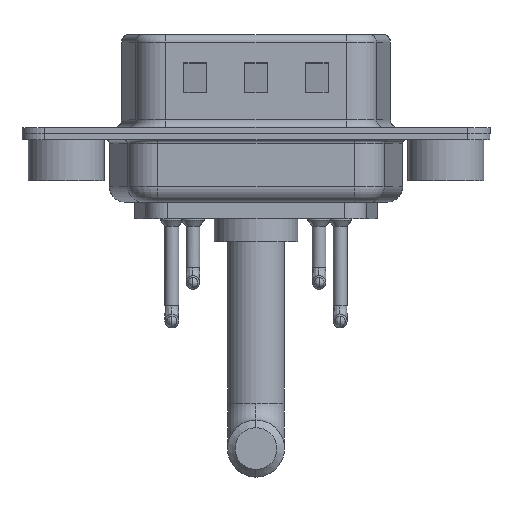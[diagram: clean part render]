
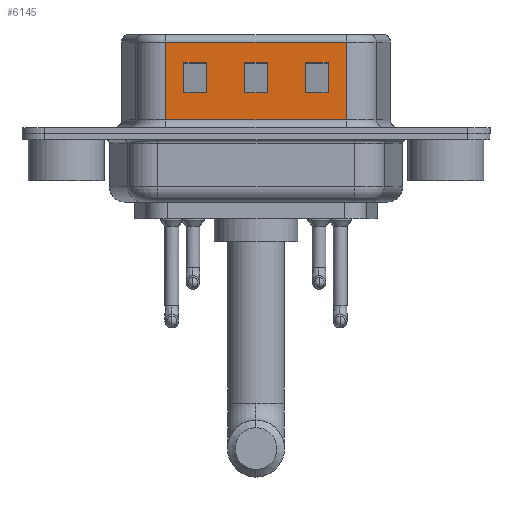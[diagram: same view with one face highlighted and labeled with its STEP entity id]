
A CAD part, front view. The second image highlights one B-rep face of the part: STEP entity #6145.
In plain terms, the highlighted planar face has unit normal (0, -1, 0).
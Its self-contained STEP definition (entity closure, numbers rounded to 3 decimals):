
#58 = VECTOR ( 'NONE', #6929, 1000. ) ;
#117 = AXIS2_PLACEMENT_3D ( 'NONE', #632, #735, #10937 ) ;
#134 = VECTOR ( 'NONE', #10615, 1000. ) ;
#245 = CARTESIAN_POINT ( 'NONE',  ( 18.451, -4.55, 6.02 ) ) ;
#406 = CARTESIAN_POINT ( 'NONE',  ( 13.25, -4.55, 4.705 ) ) ;
#409 = LINE ( 'NONE', #6395, #10310 ) ;
#414 = CARTESIAN_POINT ( 'NONE',  ( 6.549, -4.55, 0.9 ) ) ;
#632 = CARTESIAN_POINT ( 'NONE',  ( 18.451, -4.55, 6.52 ) ) ;
#735 = DIRECTION ( 'NONE',  ( 0., 1., 0. ) ) ;
#1160 = LINE ( 'NONE', #11468, #15240 ) ;
#1430 = ORIENTED_EDGE ( 'NONE', *, *, #16642, .T. ) ;
#1433 = EDGE_CURVE ( 'NONE', #14600, #17532, #16734, .T. ) ;
#1516 = CARTESIAN_POINT ( 'NONE',  ( 18.451, -4.55, 0.9 ) ) ;
#1538 = CARTESIAN_POINT ( 'NONE',  ( 13.25, -4.55, 6.52 ) ) ;
#1655 = EDGE_LOOP ( 'NONE', ( #2339, #8124, #1430, #2945 ) ) ;
#1727 = CARTESIAN_POINT ( 'NONE',  ( 22.451, -4.55, 4.705 ) ) ;
#1735 = DIRECTION ( 'NONE',  ( -1., 0., 0. ) ) ;
#1868 = VERTEX_POINT ( 'NONE', #414 ) ;
#2016 = PLANE ( 'NONE',  #117 ) ;
#2027 = EDGE_LOOP ( 'NONE', ( #11961, #11891, #10705, #10154 ) ) ;
#2086 = CARTESIAN_POINT ( 'NONE',  ( 11.75, -4.55, 2.705 ) ) ;
#2339 = ORIENTED_EDGE ( 'NONE', *, *, #18129, .T. ) ;
#2393 = CARTESIAN_POINT ( 'NONE',  ( 18.451, -4.55, 0.9 ) ) ;
#2700 = CARTESIAN_POINT ( 'NONE',  ( 15.75, -4.55, 4.705 ) ) ;
#2804 = CARTESIAN_POINT ( 'NONE',  ( 15.75, -4.55, 6.52 ) ) ;
#2911 = VERTEX_POINT ( 'NONE', #2700 ) ;
#2945 = ORIENTED_EDGE ( 'NONE', *, *, #7511, .T. ) ;
#3019 = VECTOR ( 'NONE', #12900, 1000. ) ;
#3133 = DIRECTION ( 'NONE',  ( 0., 0., 1. ) ) ;
#3438 = DIRECTION ( 'NONE',  ( 0., 0., 1. ) ) ;
#3482 = LINE ( 'NONE', #1727, #17855 ) ;
#3500 = EDGE_LOOP ( 'NONE', ( #7476, #10451, #7581, #7865 ) ) ;
#3657 = VERTEX_POINT ( 'NONE', #11320 ) ;
#3821 = EDGE_CURVE ( 'NONE', #17739, #10641, #14548, .T. ) ;
#3990 = VECTOR ( 'NONE', #15530, 1000. ) ;
#4045 = EDGE_CURVE ( 'NONE', #10447, #2911, #18175, .T. ) ;
#4546 = LINE ( 'NONE', #4635, #134 ) ;
#4635 = CARTESIAN_POINT ( 'NONE',  ( 17.25, -4.55, 6.52 ) ) ;
#4716 = VECTOR ( 'NONE', #1735, 1000. ) ;
#5061 = FACE_BOUND ( 'NONE', #3500, .T. ) ;
#5177 = CARTESIAN_POINT ( 'NONE',  ( 18.451, -4.55, 4.705 ) ) ;
#5260 = EDGE_CURVE ( 'NONE', #1868, #14274, #16618, .T. ) ;
#5423 = VERTEX_POINT ( 'NONE', #2086 ) ;
#6145 = ADVANCED_FACE ( 'NONE', ( #17207, #5061, #14047, #6521 ), #2016, .F. ) ;
#6224 = DIRECTION ( 'NONE',  ( 1., 0., 0. ) ) ;
#6346 = VERTEX_POINT ( 'NONE', #8486 ) ;
#6395 = CARTESIAN_POINT ( 'NONE',  ( 14.451, -4.55, 4.705 ) ) ;
#6442 = VERTEX_POINT ( 'NONE', #13268 ) ;
#6471 = EDGE_CURVE ( 'NONE', #18734, #11791, #4546, .T. ) ;
#6477 = VECTOR ( 'NONE', #3133, 1000. ) ;
#6521 = FACE_OUTER_BOUND ( 'NONE', #10357, .T. ) ;
#6570 = CARTESIAN_POINT ( 'NONE',  ( 15.75, -4.55, 2.705 ) ) ;
#6929 = DIRECTION ( 'NONE',  ( -1., 0., 0. ) ) ;
#7072 = EDGE_CURVE ( 'NONE', #10641, #16116, #12359, .T. ) ;
#7476 = ORIENTED_EDGE ( 'NONE', *, *, #6471, .T. ) ;
#7511 = EDGE_CURVE ( 'NONE', #5423, #6442, #9388, .T. ) ;
#7522 = DIRECTION ( 'NONE',  ( 0., 0., -1. ) ) ;
#7578 = ORIENTED_EDGE ( 'NONE', *, *, #5260, .T. ) ;
#7581 = ORIENTED_EDGE ( 'NONE', *, *, #4045, .T. ) ;
#7796 = DIRECTION ( 'NONE',  ( 1., 0., 0. ) ) ;
#7865 = ORIENTED_EDGE ( 'NONE', *, *, #14056, .T. ) ;
#7894 = LINE ( 'NONE', #9546, #16902 ) ;
#8124 = ORIENTED_EDGE ( 'NONE', *, *, #18319, .T. ) ;
#8486 = CARTESIAN_POINT ( 'NONE',  ( 9.25, -4.55, 4.705 ) ) ;
#8517 = LINE ( 'NONE', #1538, #13091 ) ;
#8553 = EDGE_CURVE ( 'NONE', #17532, #1868, #1160, .T. ) ;
#8679 = LINE ( 'NONE', #17796, #3019 ) ;
#8778 = DIRECTION ( 'NONE',  ( 0., 0., 1. ) ) ;
#8957 = ORIENTED_EDGE ( 'NONE', *, *, #8553, .T. ) ;
#9388 = LINE ( 'NONE', #15279, #6477 ) ;
#9546 = CARTESIAN_POINT ( 'NONE',  ( 18.451, -4.55, 6.52 ) ) ;
#9547 = CARTESIAN_POINT ( 'NONE',  ( 22.451, -4.55, 2.705 ) ) ;
#9673 = DIRECTION ( 'NONE',  ( 1., 0., 0. ) ) ;
#10154 = ORIENTED_EDGE ( 'NONE', *, *, #13076, .T. ) ;
#10310 = VECTOR ( 'NONE', #12368, 1000. ) ;
#10357 = EDGE_LOOP ( 'NONE', ( #10450, #15410, #8957, #7578 ) ) ;
#10447 = VERTEX_POINT ( 'NONE', #6570 ) ;
#10450 = ORIENTED_EDGE ( 'NONE', *, *, #14114, .F. ) ;
#10451 = ORIENTED_EDGE ( 'NONE', *, *, #18701, .T. ) ;
#10615 = DIRECTION ( 'NONE',  ( 0., 0., -1. ) ) ;
#10626 = CARTESIAN_POINT ( 'NONE',  ( 7.75, -4.55, 4.705 ) ) ;
#10641 = VERTEX_POINT ( 'NONE', #13114 ) ;
#10705 = ORIENTED_EDGE ( 'NONE', *, *, #7072, .T. ) ;
#10937 = DIRECTION ( 'NONE',  ( -1., 0., 0. ) ) ;
#11050 = VECTOR ( 'NONE', #6224, 1000. ) ;
#11095 = EDGE_CURVE ( 'NONE', #6346, #17739, #8679, .T. ) ;
#11320 = CARTESIAN_POINT ( 'NONE',  ( 13.25, -4.55, 2.705 ) ) ;
#11468 = CARTESIAN_POINT ( 'NONE',  ( 6.549, -4.55, 6.52 ) ) ;
#11667 = DIRECTION ( 'NONE',  ( 0., 0., -1. ) ) ;
#11791 = VERTEX_POINT ( 'NONE', #15504 ) ;
#11805 = CARTESIAN_POINT ( 'NONE',  ( 6.549, -4.55, 6.02 ) ) ;
#11891 = ORIENTED_EDGE ( 'NONE', *, *, #3821, .T. ) ;
#11961 = ORIENTED_EDGE ( 'NONE', *, *, #11095, .T. ) ;
#12359 = LINE ( 'NONE', #12443, #18044 ) ;
#12368 = DIRECTION ( 'NONE',  ( 1., 0., 0. ) ) ;
#12443 = CARTESIAN_POINT ( 'NONE',  ( 7.75, -4.55, 6.52 ) ) ;
#12546 = CARTESIAN_POINT ( 'NONE',  ( 18.451, -4.55, 2.705 ) ) ;
#12900 = DIRECTION ( 'NONE',  ( 0., 0., -1. ) ) ;
#13076 = EDGE_CURVE ( 'NONE', #16116, #6346, #409, .T. ) ;
#13091 = VECTOR ( 'NONE', #7522, 1000. ) ;
#13114 = CARTESIAN_POINT ( 'NONE',  ( 7.75, -4.55, 2.705 ) ) ;
#13268 = CARTESIAN_POINT ( 'NONE',  ( 11.75, -4.55, 4.705 ) ) ;
#13485 = VECTOR ( 'NONE', #15588, 1000. ) ;
#14038 = DIRECTION ( 'NONE',  ( 0., 0., -1. ) ) ;
#14047 = FACE_BOUND ( 'NONE', #1655, .T. ) ;
#14056 = EDGE_CURVE ( 'NONE', #2911, #18734, #3482, .T. ) ;
#14072 = LINE ( 'NONE', #5177, #19043 ) ;
#14114 = EDGE_CURVE ( 'NONE', #14600, #14274, #7894, .T. ) ;
#14145 = CARTESIAN_POINT ( 'NONE',  ( 17.25, -4.55, 4.705 ) ) ;
#14274 = VERTEX_POINT ( 'NONE', #2393 ) ;
#14548 = LINE ( 'NONE', #19064, #58 ) ;
#14600 = VERTEX_POINT ( 'NONE', #15892 ) ;
#15240 = VECTOR ( 'NONE', #11667, 1000. ) ;
#15279 = CARTESIAN_POINT ( 'NONE',  ( 11.75, -4.55, 6.52 ) ) ;
#15410 = ORIENTED_EDGE ( 'NONE', *, *, #1433, .T. ) ;
#15411 = LINE ( 'NONE', #12546, #13485 ) ;
#15504 = CARTESIAN_POINT ( 'NONE',  ( 17.25, -4.55, 2.705 ) ) ;
#15530 = DIRECTION ( 'NONE',  ( -1., 0., 0. ) ) ;
#15588 = DIRECTION ( 'NONE',  ( -1., 0., 0. ) ) ;
#15892 = CARTESIAN_POINT ( 'NONE',  ( 18.451, -4.55, 6.02 ) ) ;
#16050 = VECTOR ( 'NONE', #8778, 1000. ) ;
#16116 = VERTEX_POINT ( 'NONE', #10626 ) ;
#16618 = LINE ( 'NONE', #1516, #11050 ) ;
#16642 = EDGE_CURVE ( 'NONE', #3657, #5423, #15411, .T. ) ;
#16697 = VERTEX_POINT ( 'NONE', #406 ) ;
#16734 = LINE ( 'NONE', #245, #4716 ) ;
#16902 = VECTOR ( 'NONE', #14038, 1000. ) ;
#16994 = CARTESIAN_POINT ( 'NONE',  ( 9.25, -4.55, 2.705 ) ) ;
#17207 = FACE_BOUND ( 'NONE', #2027, .T. ) ;
#17532 = VERTEX_POINT ( 'NONE', #11805 ) ;
#17739 = VERTEX_POINT ( 'NONE', #16994 ) ;
#17796 = CARTESIAN_POINT ( 'NONE',  ( 9.25, -4.55, 6.52 ) ) ;
#17855 = VECTOR ( 'NONE', #7796, 1000. ) ;
#18044 = VECTOR ( 'NONE', #3438, 1000. ) ;
#18129 = EDGE_CURVE ( 'NONE', #6442, #16697, #14072, .T. ) ;
#18175 = LINE ( 'NONE', #2804, #16050 ) ;
#18287 = LINE ( 'NONE', #9547, #3990 ) ;
#18319 = EDGE_CURVE ( 'NONE', #16697, #3657, #8517, .T. ) ;
#18701 = EDGE_CURVE ( 'NONE', #11791, #10447, #18287, .T. ) ;
#18734 = VERTEX_POINT ( 'NONE', #14145 ) ;
#19043 = VECTOR ( 'NONE', #9673, 1000. ) ;
#19064 = CARTESIAN_POINT ( 'NONE',  ( 14.451, -4.55, 2.705 ) ) ;
